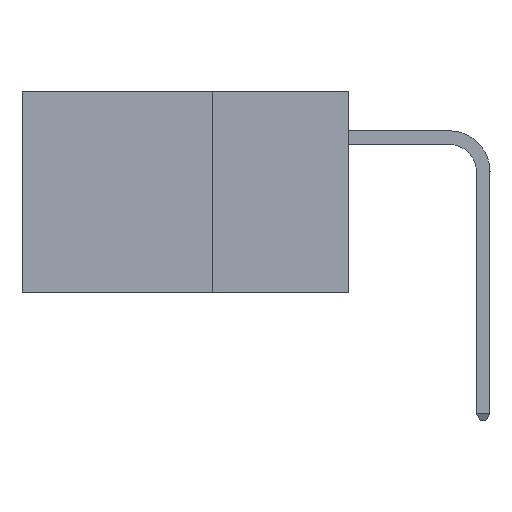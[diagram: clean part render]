
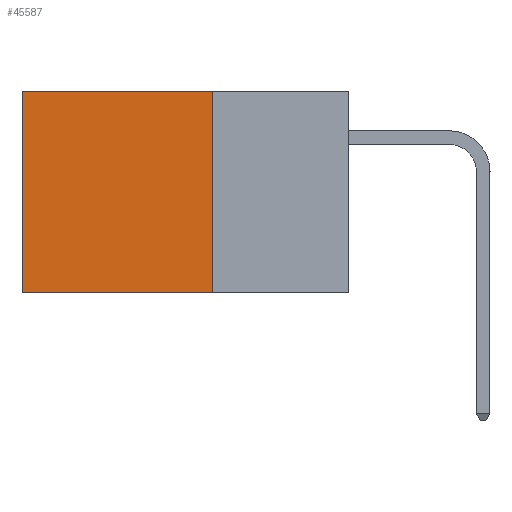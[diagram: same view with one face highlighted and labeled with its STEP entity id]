
A CAD part, left-side view. The second image highlights one B-rep face of the part: STEP entity #45587.
In plain terms, the highlighted planar face has unit normal (-1, 0, 0).
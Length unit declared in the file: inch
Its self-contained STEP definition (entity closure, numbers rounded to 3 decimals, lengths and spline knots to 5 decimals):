
#7519 = LINE ( 'NONE', #27183, #33003 ) ;
#7683 = EDGE_CURVE ( 'NONE', #31185, #50368, #7519, .T. ) ;
#8526 = DIRECTION ( 'NONE',  ( 0., 1., 0. ) ) ;
#10604 = VECTOR ( 'NONE', #8526, 39.37008 ) ;
#12149 = ORIENTED_EDGE ( 'NONE', *, *, #7683, .F. ) ;
#14087 = ORIENTED_EDGE ( 'NONE', *, *, #25538, .T. ) ;
#14955 = EDGE_LOOP ( 'NONE', ( #14087, #12149, #26862, #34769 ) ) ;
#15370 = VERTEX_POINT ( 'NONE', #43317 ) ;
#16937 = CARTESIAN_POINT ( 'NONE',  ( 0.2875, 0.6, -0.37 ) ) ;
#17117 = CARTESIAN_POINT ( 'NONE',  ( 0.2875, 0.6, 0. ) ) ;
#17291 = DIRECTION ( 'NONE',  ( 0., 0., -1. ) ) ;
#17467 = DIRECTION ( 'NONE',  ( 1., 0., 0. ) ) ;
#17792 = PLANE ( 'NONE',  #30902 ) ;
#18320 = CARTESIAN_POINT ( 'NONE',  ( 0.2875, 0.25, -0.37 ) ) ;
#20488 = CARTESIAN_POINT ( 'NONE',  ( 0.2875, 0.25, 0. ) ) ;
#21179 = LINE ( 'NONE', #20488, #10604 ) ;
#25538 = EDGE_CURVE ( 'NONE', #15370, #50368, #38338, .T. ) ;
#26531 = CARTESIAN_POINT ( 'NONE',  ( 0.2875, 0.25, 0. ) ) ;
#26862 = ORIENTED_EDGE ( 'NONE', *, *, #29297, .F. ) ;
#27183 = CARTESIAN_POINT ( 'NONE',  ( 0.2875, 0.25, -0.37 ) ) ;
#27771 = VECTOR ( 'NONE', #32604, 39.37008 ) ;
#28956 = VERTEX_POINT ( 'NONE', #35743 ) ;
#29297 = EDGE_CURVE ( 'NONE', #28956, #31185, #48468, .T. ) ;
#29982 = DIRECTION ( 'NONE',  ( 0., 0., -1. ) ) ;
#30902 = AXIS2_PLACEMENT_3D ( 'NONE', #37420, #17467, #17291 ) ;
#31185 = VERTEX_POINT ( 'NONE', #18320 ) ;
#32604 = DIRECTION ( 'NONE',  ( 0., 0., -1. ) ) ;
#33003 = VECTOR ( 'NONE', #44299, 39.37008 ) ;
#33703 = EDGE_CURVE ( 'NONE', #28956, #15370, #21179, .T. ) ;
#34769 = ORIENTED_EDGE ( 'NONE', *, *, #33703, .T. ) ;
#35560 = FACE_OUTER_BOUND ( 'NONE', #14955, .T. ) ;
#35743 = CARTESIAN_POINT ( 'NONE',  ( 0.2875, 0.25, 0. ) ) ;
#37420 = CARTESIAN_POINT ( 'NONE',  ( 0.2875, 0.25, 0. ) ) ;
#38338 = LINE ( 'NONE', #17117, #27771 ) ;
#43317 = CARTESIAN_POINT ( 'NONE',  ( 0.2875, 0.6, 0. ) ) ;
#44299 = DIRECTION ( 'NONE',  ( 0., 1., 0. ) ) ;
#45587 = ADVANCED_FACE ( 'NONE', ( #35560 ), #17792, .F. ) ;
#45947 = VECTOR ( 'NONE', #29982, 39.37008 ) ;
#48468 = LINE ( 'NONE', #26531, #45947 ) ;
#50368 = VERTEX_POINT ( 'NONE', #16937 ) ;
